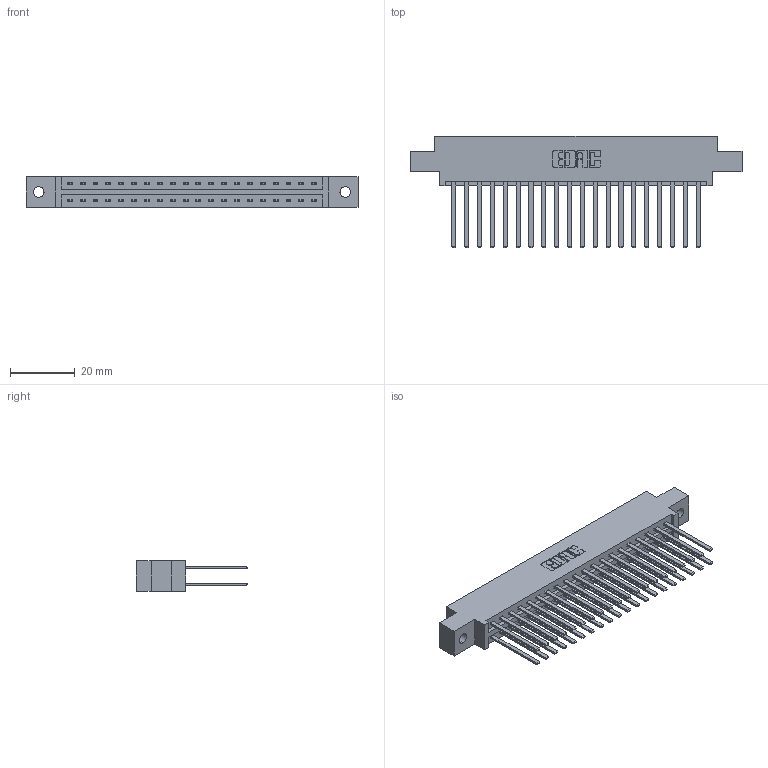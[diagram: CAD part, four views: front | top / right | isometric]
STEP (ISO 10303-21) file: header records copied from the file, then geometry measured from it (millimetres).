
FILE_DESCRIPTION (( 'STEP AP203' ), '1' );
FILE_NAME ('337-040-544-802.STEP', '2019-10-11T12:10:56', ( '' ), ( '' ), 'SwSTEP 2.0', 'SolidWorks 2016', '' );
FILE_SCHEMA (( 'CONFIG_CONTROL_DESIGN' ));
Length unit declared in the file: inch
Products named in the file (3): 345-292-001_345-293-144; 337 Part_0.170 Offset - 0.128 Dia; 337-040-544-802
Assembly tree (41 placements, depth 2):
  337-040-544-802
    337 Part_0.170 Offset - 0.128 Dia
    345-292-001_345-293-144  x40
Bounding box: 102.26 x 34.3 x 9.4 mm (x, y, z)
Volume: 10890.7 mm3; surface area: 13765.1 mm2
Topology: 41 solids, 41 shells, 2038 faces, 6043 edges, 3974 vertices
Faces by surface type: plane 1434, cylinder 604
Entity records: 18303 total; most frequent: CARTESIAN_POINT 3102, ORIENTED_EDGE 3038, DIRECTION 2675, EDGE_CURVE 1519, LINE 1395, VECTOR 1395, VERTEX_POINT 1010, AXIS2_PLACEMENT_3D 640
